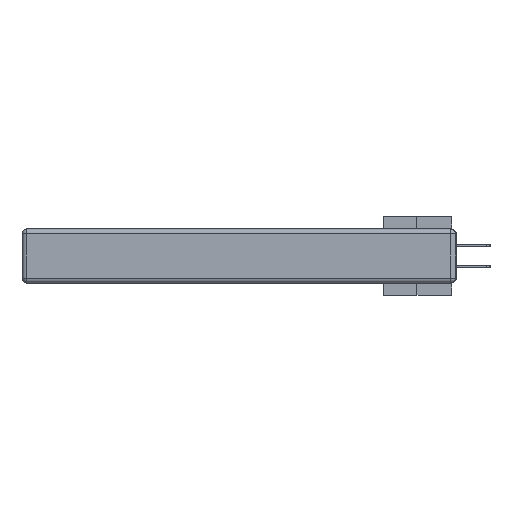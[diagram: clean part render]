
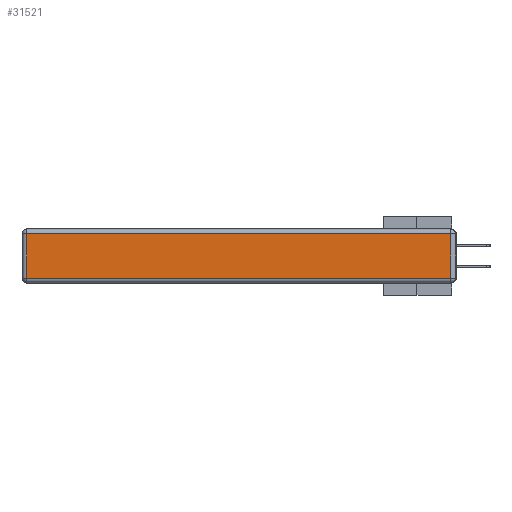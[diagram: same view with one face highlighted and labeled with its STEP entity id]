
A CAD part, left-side view. The second image highlights one B-rep face of the part: STEP entity #31521.
In plain terms, the highlighted planar face has unit normal (-1, 0, 0).
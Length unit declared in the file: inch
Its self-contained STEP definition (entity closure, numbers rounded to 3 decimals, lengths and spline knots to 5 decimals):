
#2885 = CARTESIAN_POINT ( 'NONE',  ( 0., 0.03, -0.343 ) ) ;
#3318 = DIRECTION ( 'NONE',  ( 0., 1., 0. ) ) ;
#4252 = EDGE_CURVE ( 'NONE', #4360, #30199, #28595, .T. ) ;
#4360 = VERTEX_POINT ( 'NONE', #4737 ) ;
#4709 = CARTESIAN_POINT ( 'NONE',  ( 0., 0., -0.343 ) ) ;
#4737 = CARTESIAN_POINT ( 'NONE',  ( 0., 0.03, -0.313 ) ) ;
#6372 = CARTESIAN_POINT ( 'NONE',  ( 0., 2.72, -0.03 ) ) ;
#8234 = VECTOR ( 'NONE', #32209, 39.37008 ) ;
#8907 = CARTESIAN_POINT ( 'NONE',  ( 0., 0., -0.313 ) ) ;
#8957 = VECTOR ( 'NONE', #29437, 39.37008 ) ;
#9008 = LINE ( 'NONE', #31791, #36244 ) ;
#13194 = LINE ( 'NONE', #23441, #8234 ) ;
#13378 = CARTESIAN_POINT ( 'NONE',  ( 0., 0.03, -0.03 ) ) ;
#15302 = EDGE_CURVE ( 'NONE', #30199, #36664, #9008, .T. ) ;
#16816 = VECTOR ( 'NONE', #23223, 39.37008 ) ;
#18628 = PLANE ( 'NONE',  #27191 ) ;
#18913 = ORIENTED_EDGE ( 'NONE', *, *, #27172, .T. ) ;
#22476 = CARTESIAN_POINT ( 'NONE',  ( 0., 2.72, -0.313 ) ) ;
#23223 = DIRECTION ( 'NONE',  ( 0., 0., 1. ) ) ;
#23441 = CARTESIAN_POINT ( 'NONE',  ( 0., 2.72, -0.343 ) ) ;
#23862 = ORIENTED_EDGE ( 'NONE', *, *, #4252, .T. ) ;
#27172 = EDGE_CURVE ( 'NONE', #36664, #33260, #13194, .T. ) ;
#27191 = AXIS2_PLACEMENT_3D ( 'NONE', #4709, #27207, #33214 ) ;
#27207 = DIRECTION ( 'NONE',  ( -1., 0., 0. ) ) ;
#28204 = EDGE_CURVE ( 'NONE', #33260, #4360, #33000, .T. ) ;
#28595 = LINE ( 'NONE', #2885, #16816 ) ;
#29437 = DIRECTION ( 'NONE',  ( 0., -1., 0. ) ) ;
#30199 = VERTEX_POINT ( 'NONE', #13378 ) ;
#30554 = ORIENTED_EDGE ( 'NONE', *, *, #15302, .T. ) ;
#30660 = ORIENTED_EDGE ( 'NONE', *, *, #28204, .T. ) ;
#31521 = ADVANCED_FACE ( 'NONE', ( #34597 ), #18628, .T. ) ;
#31791 = CARTESIAN_POINT ( 'NONE',  ( 0., 2.75, -0.03 ) ) ;
#32209 = DIRECTION ( 'NONE',  ( 0., 0., -1. ) ) ;
#33000 = LINE ( 'NONE', #8907, #8957 ) ;
#33214 = DIRECTION ( 'NONE',  ( 0., 0., 1. ) ) ;
#33260 = VERTEX_POINT ( 'NONE', #22476 ) ;
#34597 = FACE_OUTER_BOUND ( 'NONE', #35265, .T. ) ;
#35265 = EDGE_LOOP ( 'NONE', ( #30660, #23862, #30554, #18913 ) ) ;
#36244 = VECTOR ( 'NONE', #3318, 39.37008 ) ;
#36664 = VERTEX_POINT ( 'NONE', #6372 ) ;
